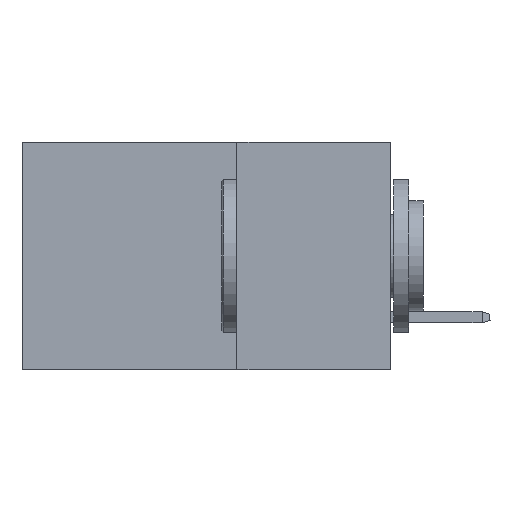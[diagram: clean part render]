
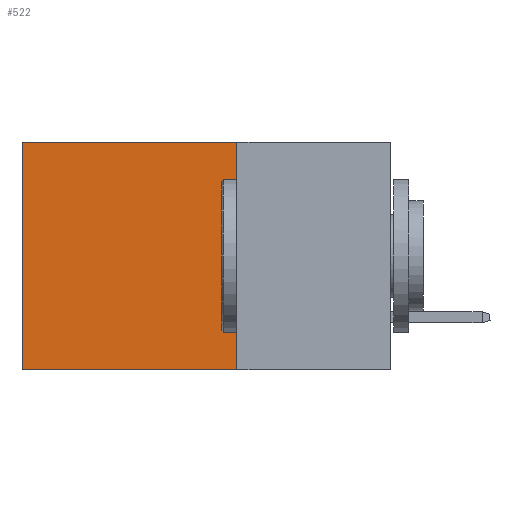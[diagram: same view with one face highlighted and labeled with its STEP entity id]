
A CAD part, left-side view. The second image highlights one B-rep face of the part: STEP entity #522.
In plain terms, the highlighted planar face has unit normal (-1, 0, 0).
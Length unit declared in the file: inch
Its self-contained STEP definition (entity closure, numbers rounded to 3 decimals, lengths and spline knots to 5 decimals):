
#522 = ADVANCED_FACE ( 'NONE', ( #5100 ), #1058, .F. ) ;
#1014 = CARTESIAN_POINT ( 'NONE',  ( 0.2875, 0.6, 0. ) ) ;
#1049 = VERTEX_POINT ( 'NONE', #7954 ) ;
#1058 = PLANE ( 'NONE',  #5965 ) ;
#1758 = VECTOR ( 'NONE', #4455, 39.37008 ) ;
#2001 = VERTEX_POINT ( 'NONE', #9407 ) ;
#2413 = DIRECTION ( 'NONE',  ( 0., 1., 0. ) ) ;
#2444 = DIRECTION ( 'NONE',  ( 0., 1., 0. ) ) ;
#2762 = CARTESIAN_POINT ( 'NONE',  ( 0.2875, 0.25, 0. ) ) ;
#2802 = DIRECTION ( 'NONE',  ( 0., 0., -1. ) ) ;
#3454 = VECTOR ( 'NONE', #2444, 39.37008 ) ;
#3464 = CARTESIAN_POINT ( 'NONE',  ( 0.2875, 0.25, 0. ) ) ;
#3694 = ORIENTED_EDGE ( 'NONE', *, *, #9472, .F. ) ;
#4369 = VECTOR ( 'NONE', #4536, 39.37008 ) ;
#4455 = DIRECTION ( 'NONE',  ( 0., 0., -1. ) ) ;
#4512 = EDGE_CURVE ( 'NONE', #6894, #2001, #9147, .T. ) ;
#4536 = DIRECTION ( 'NONE',  ( 0., 0., -1. ) ) ;
#4759 = CARTESIAN_POINT ( 'NONE',  ( 0.2875, 0.25, 0. ) ) ;
#5100 = FACE_OUTER_BOUND ( 'NONE', #8617, .T. ) ;
#5884 = EDGE_CURVE ( 'NONE', #6894, #1049, #6667, .T. ) ;
#5889 = LINE ( 'NONE', #8450, #3454 ) ;
#5965 = AXIS2_PLACEMENT_3D ( 'NONE', #2762, #7732, #2802 ) ;
#6149 = LINE ( 'NONE', #1014, #1758 ) ;
#6294 = ORIENTED_EDGE ( 'NONE', *, *, #9716, .T. ) ;
#6667 = LINE ( 'NONE', #3464, #4369 ) ;
#6894 = VERTEX_POINT ( 'NONE', #7536 ) ;
#7042 = CARTESIAN_POINT ( 'NONE',  ( 0.2875, 0.6, -0.37 ) ) ;
#7302 = ORIENTED_EDGE ( 'NONE', *, *, #4512, .T. ) ;
#7367 = VERTEX_POINT ( 'NONE', #7042 ) ;
#7536 = CARTESIAN_POINT ( 'NONE',  ( 0.2875, 0.25, 0. ) ) ;
#7732 = DIRECTION ( 'NONE',  ( 1., 0., 0. ) ) ;
#7954 = CARTESIAN_POINT ( 'NONE',  ( 0.2875, 0.25, -0.37 ) ) ;
#8450 = CARTESIAN_POINT ( 'NONE',  ( 0.2875, 0.25, -0.37 ) ) ;
#8571 = ORIENTED_EDGE ( 'NONE', *, *, #5884, .F. ) ;
#8617 = EDGE_LOOP ( 'NONE', ( #6294, #3694, #8571, #7302 ) ) ;
#8762 = VECTOR ( 'NONE', #2413, 39.37008 ) ;
#9147 = LINE ( 'NONE', #4759, #8762 ) ;
#9407 = CARTESIAN_POINT ( 'NONE',  ( 0.2875, 0.6, 0. ) ) ;
#9472 = EDGE_CURVE ( 'NONE', #1049, #7367, #5889, .T. ) ;
#9716 = EDGE_CURVE ( 'NONE', #2001, #7367, #6149, .T. ) ;
